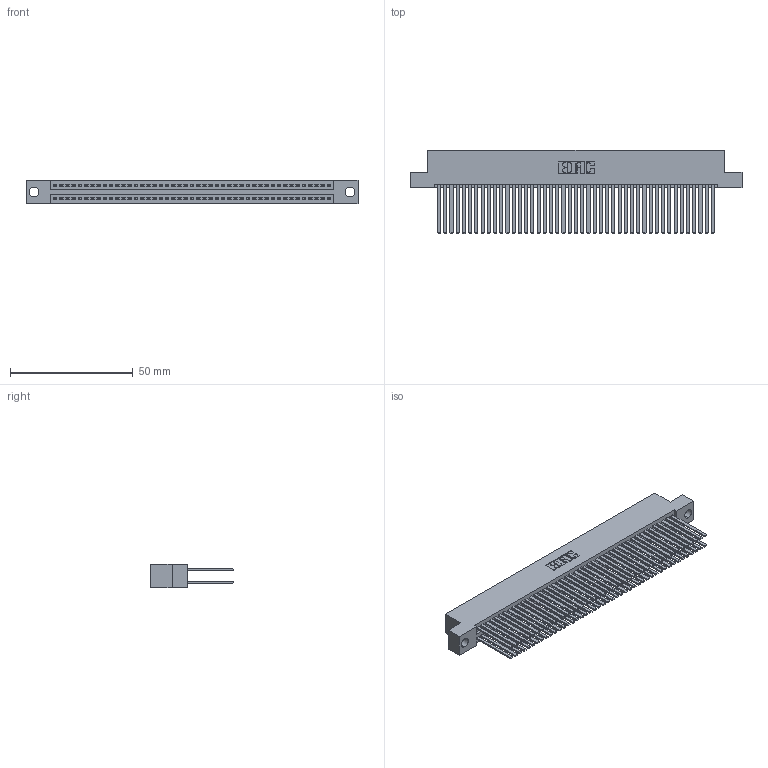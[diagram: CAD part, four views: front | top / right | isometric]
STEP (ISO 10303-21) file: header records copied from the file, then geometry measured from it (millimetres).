
FILE_DESCRIPTION (( 'STEP AP203' ), '1' );
FILE_NAME ('395-090-544-204.STEP', '2018-11-29T04:14:53', ( '' ), ( '' ), 'SwSTEP 2.0', 'SolidWorks 2016', '' );
FILE_SCHEMA (( 'CONFIG_CONTROL_DESIGN' ));
Length unit declared in the file: inch
Products named in the file (3): 345-292-001_345-293-144; 395-090-544-204; 345 Part_Flush Mounting Lugs - 0.156 Dia-TH
Assembly tree (91 placements, depth 2):
  395-090-544-204
    345 Part_Flush Mounting Lugs - 0.156 Dia-TH
    345-292-001_345-293-144  x90
Bounding box: 135.51 x 33.96 x 9.4 mm (x, y, z)
Volume: 14365.1 mm3; surface area: 24805.1 mm2
Topology: 91 solids, 91 shells, 4086 faces, 12131 edges, 7966 vertices
Faces by surface type: plane 2690, cylinder 1396
Entity records: 34723 total; most frequent: CARTESIAN_POINT 5816, ORIENTED_EDGE 5750, DIRECTION 5123, EDGE_CURVE 2875, LINE 2567, VECTOR 2567, VERTEX_POINT 1914, AXIS2_PLACEMENT_3D 1278
